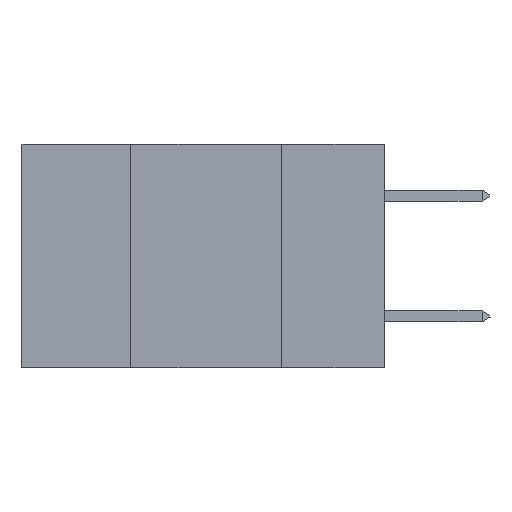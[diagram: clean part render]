
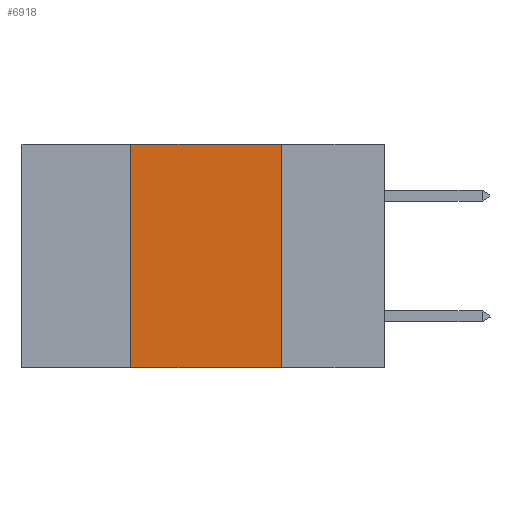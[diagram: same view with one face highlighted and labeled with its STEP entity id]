
A CAD part, left-side view. The second image highlights one B-rep face of the part: STEP entity #6918.
In plain terms, the highlighted planar face has unit normal (-1, 0, 0).
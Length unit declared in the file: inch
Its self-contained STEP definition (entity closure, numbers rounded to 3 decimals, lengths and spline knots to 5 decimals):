
#296 = VERTEX_POINT ( 'NONE', #1783 ) ;
#1439 = DIRECTION ( 'NONE',  ( 0., -1., 0. ) ) ;
#1676 = CARTESIAN_POINT ( 'NONE',  ( 0., 0.6, 0. ) ) ;
#1783 = CARTESIAN_POINT ( 'NONE',  ( 0., 0.42, 0. ) ) ;
#2457 = CARTESIAN_POINT ( 'NONE',  ( 0., 0.6, 0. ) ) ;
#2517 = VECTOR ( 'NONE', #31037, 39.37008 ) ;
#4524 = VERTEX_POINT ( 'NONE', #22686 ) ;
#5412 = VECTOR ( 'NONE', #1439, 39.37008 ) ;
#5496 = EDGE_CURVE ( 'NONE', #296, #4524, #27053, .T. ) ;
#5569 = DIRECTION ( 'NONE',  ( 0., 0., 1. ) ) ;
#6918 = ADVANCED_FACE ( 'NONE', ( #8435 ), #11418, .F. ) ;
#7098 = DIRECTION ( 'NONE',  ( 0., -1., 0. ) ) ;
#8435 = FACE_OUTER_BOUND ( 'NONE', #27315, .T. ) ;
#11412 = LINE ( 'NONE', #29505, #14088 ) ;
#11418 = PLANE ( 'NONE',  #16966 ) ;
#13527 = LINE ( 'NONE', #17011, #2517 ) ;
#14088 = VECTOR ( 'NONE', #5569, 39.37008 ) ;
#14164 = LINE ( 'NONE', #28059, #5412 ) ;
#14308 = ORIENTED_EDGE ( 'NONE', *, *, #21493, .F. ) ;
#16005 = CARTESIAN_POINT ( 'NONE',  ( 0., 0.17, -0.37 ) ) ;
#16776 = EDGE_CURVE ( 'NONE', #18046, #30349, #14164, .T. ) ;
#16966 = AXIS2_PLACEMENT_3D ( 'NONE', #1676, #28395, #20991 ) ;
#17011 = CARTESIAN_POINT ( 'NONE',  ( 0., 0.17, 0. ) ) ;
#17105 = ORIENTED_EDGE ( 'NONE', *, *, #16776, .T. ) ;
#18037 = EDGE_CURVE ( 'NONE', #4524, #30349, #13527, .T. ) ;
#18046 = VERTEX_POINT ( 'NONE', #21433 ) ;
#20854 = ORIENTED_EDGE ( 'NONE', *, *, #5496, .F. ) ;
#20991 = DIRECTION ( 'NONE',  ( 0., 0., -1. ) ) ;
#21433 = CARTESIAN_POINT ( 'NONE',  ( 0., 0.42, -0.37 ) ) ;
#21493 = EDGE_CURVE ( 'NONE', #18046, #296, #11412, .T. ) ;
#22686 = CARTESIAN_POINT ( 'NONE',  ( 0., 0.17, 0. ) ) ;
#27053 = LINE ( 'NONE', #2457, #27465 ) ;
#27315 = EDGE_LOOP ( 'NONE', ( #29248, #20854, #14308, #17105 ) ) ;
#27465 = VECTOR ( 'NONE', #7098, 39.37008 ) ;
#28059 = CARTESIAN_POINT ( 'NONE',  ( 0., 0.6, -0.37 ) ) ;
#28395 = DIRECTION ( 'NONE',  ( 1., 0., 0. ) ) ;
#29248 = ORIENTED_EDGE ( 'NONE', *, *, #18037, .F. ) ;
#29505 = CARTESIAN_POINT ( 'NONE',  ( 0., 0.42, 0. ) ) ;
#30349 = VERTEX_POINT ( 'NONE', #16005 ) ;
#31037 = DIRECTION ( 'NONE',  ( 0., 0., -1. ) ) ;
